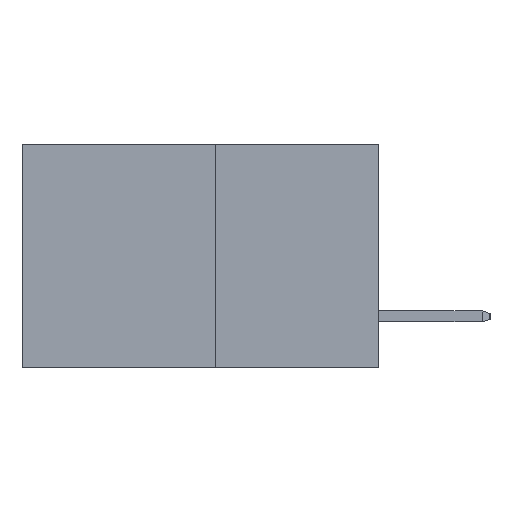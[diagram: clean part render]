
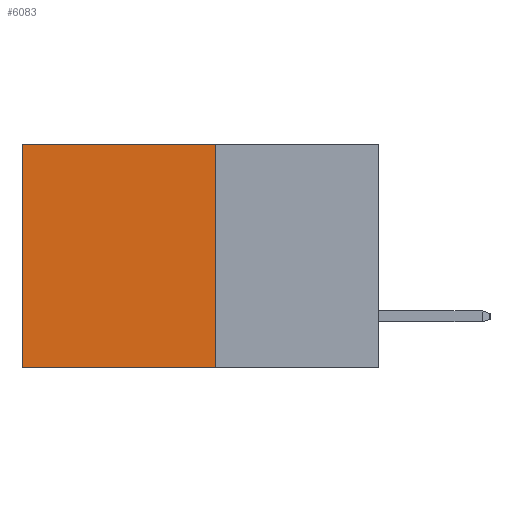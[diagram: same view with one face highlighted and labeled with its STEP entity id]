
A CAD part, left-side view. The second image highlights one B-rep face of the part: STEP entity #6083.
In plain terms, the highlighted planar face has unit normal (-1, 0, 0).
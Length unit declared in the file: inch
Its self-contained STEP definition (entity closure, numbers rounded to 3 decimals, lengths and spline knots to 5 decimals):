
#415 = VECTOR ( 'NONE', #7831, 39.37008 ) ;
#428 = CARTESIAN_POINT ( 'NONE',  ( 0.277, 0.27, -0.37 ) ) ;
#478 = VECTOR ( 'NONE', #9191, 39.37008 ) ;
#560 = EDGE_CURVE ( 'NONE', #9630, #5116, #2737, .T. ) ;
#608 = CARTESIAN_POINT ( 'NONE',  ( 0.277, 0.27, -0.37 ) ) ;
#710 = PLANE ( 'NONE',  #6329 ) ;
#1244 = EDGE_CURVE ( 'NONE', #9630, #8116, #9222, .T. ) ;
#2123 = EDGE_LOOP ( 'NONE', ( #2731, #2763, #2784, #2891 ) ) ;
#2396 = DIRECTION ( 'NONE',  ( 0., 0., -1. ) ) ;
#2480 = DIRECTION ( 'NONE',  ( 0., 0., -1. ) ) ;
#2731 = ORIENTED_EDGE ( 'NONE', *, *, #3384, .T. ) ;
#2737 = LINE ( 'NONE', #6709, #478 ) ;
#2739 = DIRECTION ( 'NONE',  ( 1., 0., 0. ) ) ;
#2763 = ORIENTED_EDGE ( 'NONE', *, *, #7382, .F. ) ;
#2784 = ORIENTED_EDGE ( 'NONE', *, *, #1244, .F. ) ;
#2891 = ORIENTED_EDGE ( 'NONE', *, *, #560, .T. ) ;
#3095 = VECTOR ( 'NONE', #4974, 39.37008 ) ;
#3384 = EDGE_CURVE ( 'NONE', #5116, #6209, #5926, .T. ) ;
#3541 = CARTESIAN_POINT ( 'NONE',  ( 0.277, 0.59, -0.37 ) ) ;
#3855 = VECTOR ( 'NONE', #2396, 39.37008 ) ;
#4974 = DIRECTION ( 'NONE',  ( 0., 0., -1. ) ) ;
#5065 = FACE_OUTER_BOUND ( 'NONE', #2123, .T. ) ;
#5116 = VERTEX_POINT ( 'NONE', #7268 ) ;
#5922 = CARTESIAN_POINT ( 'NONE',  ( 0.277, 0.27, 0. ) ) ;
#5926 = LINE ( 'NONE', #3541, #3855 ) ;
#6083 = ADVANCED_FACE ( 'NONE', ( #5065 ), #710, .F. ) ;
#6209 = VERTEX_POINT ( 'NONE', #9226 ) ;
#6329 = AXIS2_PLACEMENT_3D ( 'NONE', #428, #2739, #2480 ) ;
#6709 = CARTESIAN_POINT ( 'NONE',  ( 0.277, 0.27, 0. ) ) ;
#6762 = LINE ( 'NONE', #7126, #415 ) ;
#7126 = CARTESIAN_POINT ( 'NONE',  ( 0.277, 0.27, -0.37 ) ) ;
#7268 = CARTESIAN_POINT ( 'NONE',  ( 0.277, 0.59, 0. ) ) ;
#7271 = CARTESIAN_POINT ( 'NONE',  ( 0.277, 0.27, -0.37 ) ) ;
#7382 = EDGE_CURVE ( 'NONE', #8116, #6209, #6762, .T. ) ;
#7831 = DIRECTION ( 'NONE',  ( 0., 1., 0. ) ) ;
#8116 = VERTEX_POINT ( 'NONE', #7271 ) ;
#9191 = DIRECTION ( 'NONE',  ( 0., 1., 0. ) ) ;
#9222 = LINE ( 'NONE', #608, #3095 ) ;
#9226 = CARTESIAN_POINT ( 'NONE',  ( 0.277, 0.59, -0.37 ) ) ;
#9630 = VERTEX_POINT ( 'NONE', #5922 ) ;
